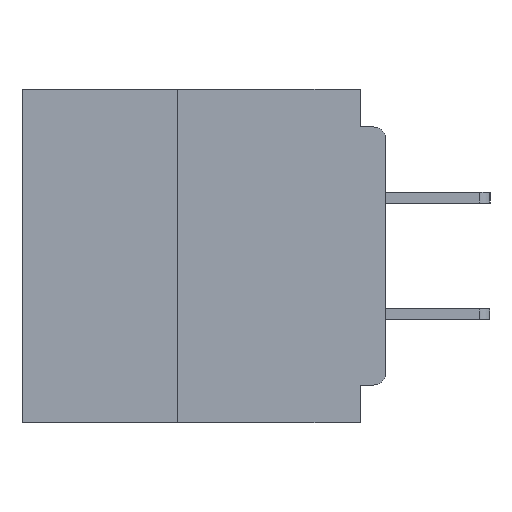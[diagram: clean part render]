
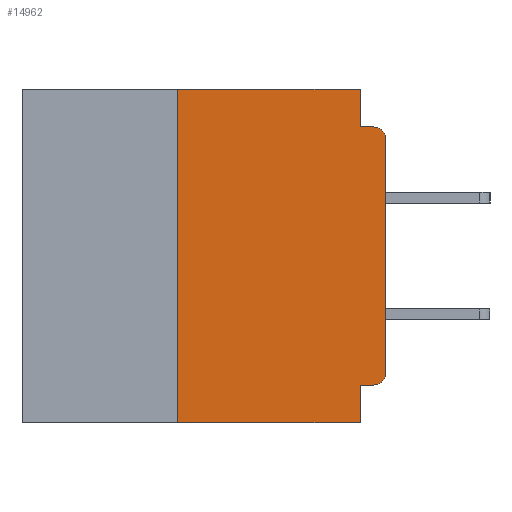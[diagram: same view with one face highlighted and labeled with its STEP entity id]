
A CAD part, left-side view. The second image highlights one B-rep face of the part: STEP entity #14962.
In plain terms, the highlighted planar face has unit normal (-1, 0, 0).
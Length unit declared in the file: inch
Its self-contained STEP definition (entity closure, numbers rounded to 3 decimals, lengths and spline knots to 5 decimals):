
#1452 = VERTEX_POINT ( 'NONE', #5727 ) ;
#1577 = EDGE_CURVE ( 'NONE', #22761, #29526, #35995, .T. ) ;
#3357 = AXIS2_PLACEMENT_3D ( 'NONE', #30706, #10292, #34162 ) ;
#3999 = VERTEX_POINT ( 'NONE', #33392 ) ;
#4159 = ORIENTED_EDGE ( 'NONE', *, *, #24163, .F. ) ;
#4413 = LINE ( 'NONE', #10071, #22624 ) ;
#4432 = CARTESIAN_POINT ( 'NONE',  ( 0., 0., 0. ) ) ;
#5121 = DIRECTION ( 'NONE',  ( 0., 0., -1. ) ) ;
#5727 = CARTESIAN_POINT ( 'NONE',  ( 0., 0.015, -0.045 ) ) ;
#6558 = DIRECTION ( 'NONE',  ( 0., 0., 1. ) ) ;
#6707 = DIRECTION ( 'NONE',  ( 0., 1., 0. ) ) ;
#9678 = AXIS2_PLACEMENT_3D ( 'NONE', #15357, #25591, #5121 ) ;
#9796 = EDGE_CURVE ( 'NONE', #20698, #1452, #10768, .T. ) ;
#10071 = CARTESIAN_POINT ( 'NONE',  ( 0., 0.437, 0. ) ) ;
#10114 = CARTESIAN_POINT ( 'NONE',  ( 0., 0.031, 0. ) ) ;
#10292 = DIRECTION ( 'NONE',  ( -1., 0., 0. ) ) ;
#10768 = LINE ( 'NONE', #43579, #38007 ) ;
#10906 = VECTOR ( 'NONE', #12226, 39.37008 ) ;
#11784 = EDGE_CURVE ( 'NONE', #40229, #1452, #18707, .T. ) ;
#11809 = VERTEX_POINT ( 'NONE', #37768 ) ;
#12226 = DIRECTION ( 'NONE',  ( 0., 0., -1. ) ) ;
#12877 = ORIENTED_EDGE ( 'NONE', *, *, #30480, .T. ) ;
#13537 = DIRECTION ( 'NONE',  ( 0., -1., 0. ) ) ;
#14962 = ADVANCED_FACE ( 'NONE', ( #40252 ), #22167, .F. ) ;
#15357 = CARTESIAN_POINT ( 'NONE',  ( 0., 0.437, 0. ) ) ;
#15479 = ORIENTED_EDGE ( 'NONE', *, *, #9796, .F. ) ;
#15615 = CARTESIAN_POINT ( 'NONE',  ( 0., 0., -0.34 ) ) ;
#16090 = ORIENTED_EDGE ( 'NONE', *, *, #35976, .F. ) ;
#16124 = VECTOR ( 'NONE', #21517, 39.37008 ) ;
#17001 = EDGE_LOOP ( 'NONE', ( #42416, #18439, #15479, #4159, #26155, #41196, #12877, #16090, #34201, #31545 ) ) ;
#18199 = LINE ( 'NONE', #37810, #25064 ) ;
#18313 = CARTESIAN_POINT ( 'NONE',  ( 0., 0., -0.06 ) ) ;
#18439 = ORIENTED_EDGE ( 'NONE', *, *, #11784, .T. ) ;
#18579 = LINE ( 'NONE', #37246, #35639 ) ;
#18617 = EDGE_CURVE ( 'NONE', #22761, #34821, #44365, .T. ) ;
#18707 = CIRCLE ( 'NONE', #3357, 0.015 ) ;
#18980 = CARTESIAN_POINT ( 'NONE',  ( 0., 0.031, -0.4 ) ) ;
#19315 = CARTESIAN_POINT ( 'NONE',  ( 0., 0.015, -0.34 ) ) ;
#20248 = DIRECTION ( 'NONE',  ( 0., 0., -1. ) ) ;
#20519 = VECTOR ( 'NONE', #6558, 39.37008 ) ;
#20698 = VERTEX_POINT ( 'NONE', #30784 ) ;
#20929 = CARTESIAN_POINT ( 'NONE',  ( 0., 0.25, -0.4 ) ) ;
#21517 = DIRECTION ( 'NONE',  ( 0., 0., 1. ) ) ;
#21912 = VERTEX_POINT ( 'NONE', #10114 ) ;
#22167 = PLANE ( 'NONE',  #9678 ) ;
#22624 = VECTOR ( 'NONE', #13537, 39.37008 ) ;
#22679 = DIRECTION ( 'NONE',  ( 0., 0., -1. ) ) ;
#22761 = VERTEX_POINT ( 'NONE', #43281 ) ;
#23169 = DIRECTION ( 'NONE',  ( 0., -1., 0. ) ) ;
#24163 = EDGE_CURVE ( 'NONE', #21912, #20698, #18579, .T. ) ;
#25064 = VECTOR ( 'NONE', #41228, 39.37008 ) ;
#25591 = DIRECTION ( 'NONE',  ( 1., 0., 0. ) ) ;
#25634 = CARTESIAN_POINT ( 'NONE',  ( 0., 0.031, -0.355 ) ) ;
#26155 = ORIENTED_EDGE ( 'NONE', *, *, #41779, .F. ) ;
#27935 = VECTOR ( 'NONE', #6707, 39.37008 ) ;
#29526 = VERTEX_POINT ( 'NONE', #25634 ) ;
#30439 = CARTESIAN_POINT ( 'NONE',  ( 0., 0.25, -0.4 ) ) ;
#30446 = CARTESIAN_POINT ( 'NONE',  ( 0., 0., -0.355 ) ) ;
#30480 = EDGE_CURVE ( 'NONE', #42534, #3999, #18199, .T. ) ;
#30706 = CARTESIAN_POINT ( 'NONE',  ( 0., 0.015, -0.06 ) ) ;
#30784 = CARTESIAN_POINT ( 'NONE',  ( 0., 0.031, -0.045 ) ) ;
#31545 = ORIENTED_EDGE ( 'NONE', *, *, #18617, .T. ) ;
#32376 = AXIS2_PLACEMENT_3D ( 'NONE', #19315, #43121, #22679 ) ;
#33392 = CARTESIAN_POINT ( 'NONE',  ( 0., 0.031, -0.4 ) ) ;
#33700 = EDGE_CURVE ( 'NONE', #42534, #11809, #38685, .T. ) ;
#34162 = DIRECTION ( 'NONE',  ( 0., 0., -1. ) ) ;
#34201 = ORIENTED_EDGE ( 'NONE', *, *, #1577, .F. ) ;
#34241 = LINE ( 'NONE', #4432, #16124 ) ;
#34821 = VERTEX_POINT ( 'NONE', #15615 ) ;
#35639 = VECTOR ( 'NONE', #20248, 39.37008 ) ;
#35976 = EDGE_CURVE ( 'NONE', #29526, #3999, #38152, .T. ) ;
#35995 = LINE ( 'NONE', #30446, #27935 ) ;
#37246 = CARTESIAN_POINT ( 'NONE',  ( 0., 0.031, 0. ) ) ;
#37768 = CARTESIAN_POINT ( 'NONE',  ( 0., 0.25, 0. ) ) ;
#37810 = CARTESIAN_POINT ( 'NONE',  ( 0., 0.437, -0.4 ) ) ;
#38007 = VECTOR ( 'NONE', #23169, 39.37008 ) ;
#38152 = LINE ( 'NONE', #18980, #10906 ) ;
#38685 = LINE ( 'NONE', #30439, #20519 ) ;
#40229 = VERTEX_POINT ( 'NONE', #18313 ) ;
#40252 = FACE_OUTER_BOUND ( 'NONE', #17001, .T. ) ;
#41196 = ORIENTED_EDGE ( 'NONE', *, *, #33700, .F. ) ;
#41228 = DIRECTION ( 'NONE',  ( 0., -1., 0. ) ) ;
#41779 = EDGE_CURVE ( 'NONE', #11809, #21912, #4413, .T. ) ;
#42416 = ORIENTED_EDGE ( 'NONE', *, *, #43236, .T. ) ;
#42534 = VERTEX_POINT ( 'NONE', #20929 ) ;
#43121 = DIRECTION ( 'NONE',  ( -1., 0., 0. ) ) ;
#43236 = EDGE_CURVE ( 'NONE', #34821, #40229, #34241, .T. ) ;
#43281 = CARTESIAN_POINT ( 'NONE',  ( 0., 0.015, -0.355 ) ) ;
#43579 = CARTESIAN_POINT ( 'NONE',  ( 0., 0., -0.045 ) ) ;
#44365 = CIRCLE ( 'NONE', #32376, 0.015 ) ;
